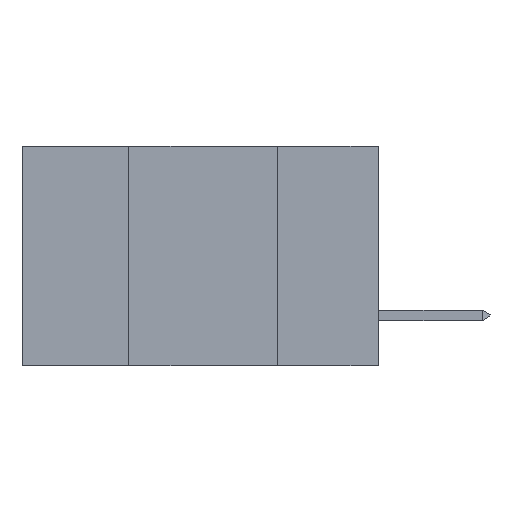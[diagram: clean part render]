
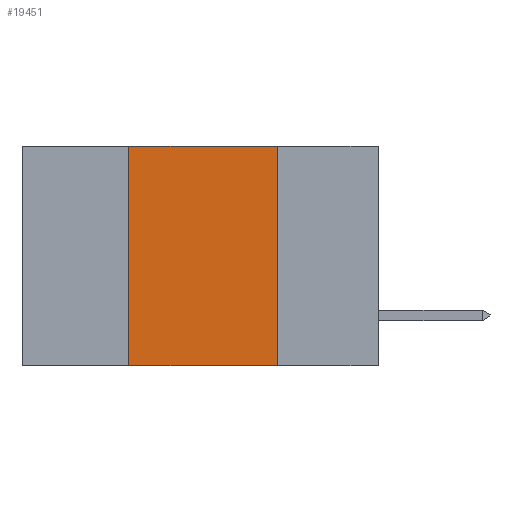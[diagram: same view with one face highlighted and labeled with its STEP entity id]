
A CAD part, left-side view. The second image highlights one B-rep face of the part: STEP entity #19451.
In plain terms, the highlighted planar face has unit normal (-1, 0, 0).
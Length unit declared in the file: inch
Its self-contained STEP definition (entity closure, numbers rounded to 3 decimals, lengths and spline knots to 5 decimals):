
#1324 = ORIENTED_EDGE ( 'NONE', *, *, #5430, .F. ) ;
#1811 = CARTESIAN_POINT ( 'NONE',  ( 0., 0.17, -0.37 ) ) ;
#2636 = VERTEX_POINT ( 'NONE', #10816 ) ;
#3499 = ORIENTED_EDGE ( 'NONE', *, *, #6208, .F. ) ;
#4329 = DIRECTION ( 'NONE',  ( 0., 0., 1. ) ) ;
#4489 = EDGE_CURVE ( 'NONE', #2636, #12377, #17549, .T. ) ;
#5094 = DIRECTION ( 'NONE',  ( 0., -1., 0. ) ) ;
#5430 = EDGE_CURVE ( 'NONE', #2636, #12504, #14619, .T. ) ;
#6172 = FACE_OUTER_BOUND ( 'NONE', #7306, .T. ) ;
#6208 = EDGE_CURVE ( 'NONE', #12504, #12214, #14222, .T. ) ;
#6372 = VECTOR ( 'NONE', #13080, 39.37008 ) ;
#7306 = EDGE_LOOP ( 'NONE', ( #18862, #3499, #1324, #17404 ) ) ;
#7550 = DIRECTION ( 'NONE',  ( 1., 0., 0. ) ) ;
#7662 = CARTESIAN_POINT ( 'NONE',  ( 0., 0.6, 0. ) ) ;
#7856 = CARTESIAN_POINT ( 'NONE',  ( 0., 0.42, 0. ) ) ;
#9345 = EDGE_CURVE ( 'NONE', #12214, #12377, #21878, .T. ) ;
#9566 = VECTOR ( 'NONE', #10586, 39.37008 ) ;
#10586 = DIRECTION ( 'NONE',  ( 0., -1., 0. ) ) ;
#10792 = CARTESIAN_POINT ( 'NONE',  ( 0., 0.6, 0. ) ) ;
#10816 = CARTESIAN_POINT ( 'NONE',  ( 0., 0.42, -0.37 ) ) ;
#12214 = VERTEX_POINT ( 'NONE', #20111 ) ;
#12315 = AXIS2_PLACEMENT_3D ( 'NONE', #7662, #7550, #19745 ) ;
#12377 = VERTEX_POINT ( 'NONE', #1811 ) ;
#12504 = VERTEX_POINT ( 'NONE', #7856 ) ;
#13080 = DIRECTION ( 'NONE',  ( 0., 0., -1. ) ) ;
#13900 = CARTESIAN_POINT ( 'NONE',  ( 0., 0.6, -0.37 ) ) ;
#14222 = LINE ( 'NONE', #10792, #16177 ) ;
#14619 = LINE ( 'NONE', #19963, #21614 ) ;
#16177 = VECTOR ( 'NONE', #5094, 39.37008 ) ;
#16963 = CARTESIAN_POINT ( 'NONE',  ( 0., 0.17, -0.37 ) ) ;
#17404 = ORIENTED_EDGE ( 'NONE', *, *, #4489, .T. ) ;
#17549 = LINE ( 'NONE', #13900, #9566 ) ;
#18037 = PLANE ( 'NONE',  #12315 ) ;
#18862 = ORIENTED_EDGE ( 'NONE', *, *, #9345, .F. ) ;
#19451 = ADVANCED_FACE ( 'NONE', ( #6172 ), #18037, .F. ) ;
#19745 = DIRECTION ( 'NONE',  ( 0., 0., -1. ) ) ;
#19963 = CARTESIAN_POINT ( 'NONE',  ( 0., 0.42, -0.37 ) ) ;
#20111 = CARTESIAN_POINT ( 'NONE',  ( 0., 0.17, 0. ) ) ;
#21614 = VECTOR ( 'NONE', #4329, 39.37008 ) ;
#21878 = LINE ( 'NONE', #16963, #6372 ) ;
